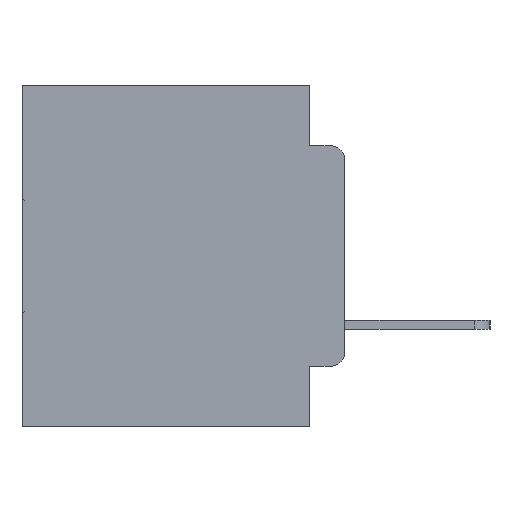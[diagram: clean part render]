
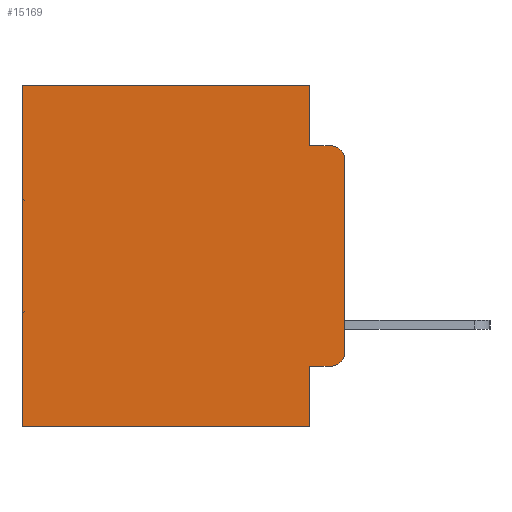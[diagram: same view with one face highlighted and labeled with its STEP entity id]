
A CAD part, left-side view. The second image highlights one B-rep face of the part: STEP entity #15169.
In plain terms, the highlighted planar face has unit normal (-1, 0, 0).
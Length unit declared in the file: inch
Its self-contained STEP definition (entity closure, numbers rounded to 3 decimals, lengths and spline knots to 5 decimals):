
#589 = DIRECTION ( 'NONE',  ( 0., 0., -1. ) ) ;
#811 = AXIS2_PLACEMENT_3D ( 'NONE', #30102, #16173, #589 ) ;
#1375 = VERTEX_POINT ( 'NONE', #23779 ) ;
#2101 = CARTESIAN_POINT ( 'NONE',  ( 0.298, 0.02, -0.4115 ) ) ;
#2107 = EDGE_CURVE ( 'NONE', #21382, #21115, #29693, .T. ) ;
#2553 = DIRECTION ( 'NONE',  ( 0., 0., -1. ) ) ;
#2959 = ORIENTED_EDGE ( 'NONE', *, *, #26004, .F. ) ;
#3403 = VECTOR ( 'NONE', #9417, 39.37008 ) ;
#3879 = LINE ( 'NONE', #26239, #9954 ) ;
#4552 = FACE_OUTER_BOUND ( 'NONE', #21850, .T. ) ;
#4644 = LINE ( 'NONE', #30098, #29747 ) ;
#5245 = LINE ( 'NONE', #23072, #11293 ) ;
#5547 = CIRCLE ( 'NONE', #811, 0.02 ) ;
#5655 = DIRECTION ( 'NONE',  ( 0., -1., 0. ) ) ;
#6050 = AXIS2_PLACEMENT_3D ( 'NONE', #29464, #17966, #2553 ) ;
#7720 = CARTESIAN_POINT ( 'NONE',  ( 0.298, 0.051, -0.0885 ) ) ;
#8022 = EDGE_CURVE ( 'NONE', #14292, #21115, #5547, .T. ) ;
#9417 = DIRECTION ( 'NONE',  ( 0., 1., 0. ) ) ;
#9876 = ORIENTED_EDGE ( 'NONE', *, *, #24491, .F. ) ;
#9954 = VECTOR ( 'NONE', #30904, 39.37008 ) ;
#10104 = CARTESIAN_POINT ( 'NONE',  ( 0.298, 0.051, 0. ) ) ;
#10282 = LINE ( 'NONE', #21766, #3403 ) ;
#10882 = VERTEX_POINT ( 'NONE', #12789 ) ;
#11293 = VECTOR ( 'NONE', #5655, 39.37008 ) ;
#11458 = EDGE_CURVE ( 'NONE', #10882, #14292, #5245, .T. ) ;
#12092 = CARTESIAN_POINT ( 'NONE',  ( 0.298, 0.473, 0. ) ) ;
#12277 = ORIENTED_EDGE ( 'NONE', *, *, #13192, .F. ) ;
#12495 = VECTOR ( 'NONE', #19690, 39.37008 ) ;
#12789 = CARTESIAN_POINT ( 'NONE',  ( 0.298, 0.051, -0.4115 ) ) ;
#12872 = PLANE ( 'NONE',  #6050 ) ;
#13192 = EDGE_CURVE ( 'NONE', #10882, #31866, #3879, .T. ) ;
#13220 = CARTESIAN_POINT ( 'NONE',  ( 0.298, 0.02, -0.1085 ) ) ;
#13316 = LINE ( 'NONE', #12092, #12495 ) ;
#13460 = AXIS2_PLACEMENT_3D ( 'NONE', #13220, #29736, #15771 ) ;
#13514 = CARTESIAN_POINT ( 'NONE',  ( 0.298, 0.473, -0.5 ) ) ;
#13633 = DIRECTION ( 'NONE',  ( 0., -1., 0. ) ) ;
#13753 = CARTESIAN_POINT ( 'NONE',  ( 0.298, 0., -0.5 ) ) ;
#13853 = VERTEX_POINT ( 'NONE', #10104 ) ;
#13861 = LINE ( 'NONE', #13753, #25778 ) ;
#14286 = ORIENTED_EDGE ( 'NONE', *, *, #2107, .F. ) ;
#14292 = VERTEX_POINT ( 'NONE', #2101 ) ;
#14371 = VERTEX_POINT ( 'NONE', #7720 ) ;
#15169 = ADVANCED_FACE ( 'NONE', ( #4552 ), #12872, .F. ) ;
#15771 = DIRECTION ( 'NONE',  ( 0., 0., -1. ) ) ;
#15870 = ORIENTED_EDGE ( 'NONE', *, *, #27537, .T. ) ;
#16173 = DIRECTION ( 'NONE',  ( -1., 0., 0. ) ) ;
#16290 = DIRECTION ( 'NONE',  ( 0., 1., 0. ) ) ;
#16584 = EDGE_CURVE ( 'NONE', #21327, #21762, #13316, .T. ) ;
#17152 = CARTESIAN_POINT ( 'NONE',  ( 0.298, 0., 0. ) ) ;
#17300 = CARTESIAN_POINT ( 'NONE',  ( 0.298, 0.473, 0. ) ) ;
#17469 = ORIENTED_EDGE ( 'NONE', *, *, #27186, .T. ) ;
#17966 = DIRECTION ( 'NONE',  ( 1., 0., 0. ) ) ;
#19119 = CARTESIAN_POINT ( 'NONE',  ( 0.298, 0., -0.3915 ) ) ;
#19170 = CARTESIAN_POINT ( 'NONE',  ( 0.298, 0.051, 0. ) ) ;
#19690 = DIRECTION ( 'NONE',  ( 0., 0., -1. ) ) ;
#20211 = VECTOR ( 'NONE', #25993, 39.37008 ) ;
#21115 = VERTEX_POINT ( 'NONE', #19119 ) ;
#21327 = VERTEX_POINT ( 'NONE', #17300 ) ;
#21382 = VERTEX_POINT ( 'NONE', #26644 ) ;
#21762 = VERTEX_POINT ( 'NONE', #13514 ) ;
#21766 = CARTESIAN_POINT ( 'NONE',  ( 0.298, 0., 0. ) ) ;
#21850 = EDGE_LOOP ( 'NONE', ( #14286, #15870, #2959, #9876, #17469, #29729, #30432, #12277, #24067, #30810 ) ) ;
#23072 = CARTESIAN_POINT ( 'NONE',  ( 0.298, 0.051, -0.4115 ) ) ;
#23652 = VECTOR ( 'NONE', #30486, 39.37008 ) ;
#23692 = CIRCLE ( 'NONE', #13460, 0.02 ) ;
#23779 = CARTESIAN_POINT ( 'NONE',  ( 0.298, 0.02, -0.0885 ) ) ;
#24067 = ORIENTED_EDGE ( 'NONE', *, *, #11458, .T. ) ;
#24491 = EDGE_CURVE ( 'NONE', #13853, #14371, #27004, .T. ) ;
#25778 = VECTOR ( 'NONE', #16290, 39.37008 ) ;
#25993 = DIRECTION ( 'NONE',  ( 0., 0., -1. ) ) ;
#26004 = EDGE_CURVE ( 'NONE', #14371, #1375, #4644, .T. ) ;
#26239 = CARTESIAN_POINT ( 'NONE',  ( 0.298, 0.051, 0. ) ) ;
#26389 = CARTESIAN_POINT ( 'NONE',  ( 0.298, 0.051, -0.5 ) ) ;
#26644 = CARTESIAN_POINT ( 'NONE',  ( 0.298, 0., -0.1085 ) ) ;
#27004 = LINE ( 'NONE', #19170, #20211 ) ;
#27186 = EDGE_CURVE ( 'NONE', #13853, #21327, #10282, .T. ) ;
#27537 = EDGE_CURVE ( 'NONE', #21382, #1375, #23692, .T. ) ;
#27948 = EDGE_CURVE ( 'NONE', #31866, #21762, #13861, .T. ) ;
#29464 = CARTESIAN_POINT ( 'NONE',  ( 0.298, 0., 0. ) ) ;
#29693 = LINE ( 'NONE', #17152, #23652 ) ;
#29729 = ORIENTED_EDGE ( 'NONE', *, *, #16584, .T. ) ;
#29736 = DIRECTION ( 'NONE',  ( -1., 0., 0. ) ) ;
#29747 = VECTOR ( 'NONE', #13633, 39.37008 ) ;
#30098 = CARTESIAN_POINT ( 'NONE',  ( 0.298, 0.051, -0.0885 ) ) ;
#30102 = CARTESIAN_POINT ( 'NONE',  ( 0.298, 0.02, -0.3915 ) ) ;
#30432 = ORIENTED_EDGE ( 'NONE', *, *, #27948, .F. ) ;
#30486 = DIRECTION ( 'NONE',  ( 0., 0., -1. ) ) ;
#30810 = ORIENTED_EDGE ( 'NONE', *, *, #8022, .T. ) ;
#30904 = DIRECTION ( 'NONE',  ( 0., 0., -1. ) ) ;
#31866 = VERTEX_POINT ( 'NONE', #26389 ) ;
